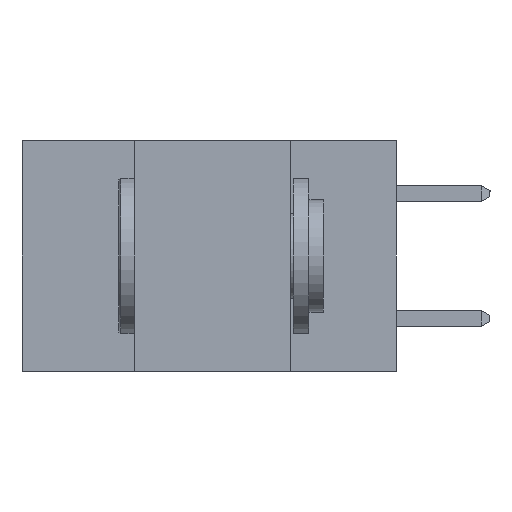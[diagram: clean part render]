
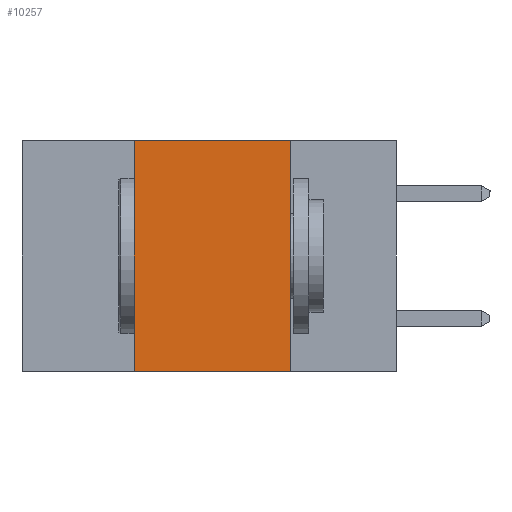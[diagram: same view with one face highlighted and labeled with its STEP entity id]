
A CAD part, left-side view. The second image highlights one B-rep face of the part: STEP entity #10257.
In plain terms, the highlighted planar face has unit normal (-1, 0, 0).
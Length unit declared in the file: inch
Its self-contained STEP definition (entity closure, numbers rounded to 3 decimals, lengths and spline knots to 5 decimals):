
#478 = CARTESIAN_POINT ( 'NONE',  ( 0., 0.6, -0.37 ) ) ;
#759 = DIRECTION ( 'NONE',  ( 0., 0., -1. ) ) ;
#1165 = LINE ( 'NONE', #14763, #4010 ) ;
#1431 = VERTEX_POINT ( 'NONE', #18993 ) ;
#2068 = ORIENTED_EDGE ( 'NONE', *, *, #12775, .T. ) ;
#2248 = VERTEX_POINT ( 'NONE', #3131 ) ;
#3131 = CARTESIAN_POINT ( 'NONE',  ( 0., 0.42, 0. ) ) ;
#4010 = VECTOR ( 'NONE', #21009, 39.37008 ) ;
#4661 = VECTOR ( 'NONE', #16348, 39.37008 ) ;
#5045 = DIRECTION ( 'NONE',  ( 0., 0., -1. ) ) ;
#5070 = EDGE_CURVE ( 'NONE', #1431, #13845, #5148, .T. ) ;
#5087 = CARTESIAN_POINT ( 'NONE',  ( 0., 0.42, -0.37 ) ) ;
#5148 = LINE ( 'NONE', #16434, #9303 ) ;
#5977 = PLANE ( 'NONE',  #16750 ) ;
#6089 = EDGE_CURVE ( 'NONE', #10722, #2248, #13156, .T. ) ;
#8229 = DIRECTION ( 'NONE',  ( 0., 0., 1. ) ) ;
#8542 = EDGE_LOOP ( 'NONE', ( #10098, #16438, #9071, #2068 ) ) ;
#8891 = FACE_OUTER_BOUND ( 'NONE', #8542, .T. ) ;
#8998 = DIRECTION ( 'NONE',  ( 1., 0., 0. ) ) ;
#9071 = ORIENTED_EDGE ( 'NONE', *, *, #6089, .F. ) ;
#9303 = VECTOR ( 'NONE', #5045, 39.37008 ) ;
#10098 = ORIENTED_EDGE ( 'NONE', *, *, #5070, .F. ) ;
#10257 = ADVANCED_FACE ( 'NONE', ( #8891 ), #5977, .F. ) ;
#10722 = VERTEX_POINT ( 'NONE', #14125 ) ;
#12775 = EDGE_CURVE ( 'NONE', #10722, #13845, #13554, .T. ) ;
#13156 = LINE ( 'NONE', #5087, #14172 ) ;
#13554 = LINE ( 'NONE', #478, #4661 ) ;
#13845 = VERTEX_POINT ( 'NONE', #15716 ) ;
#14125 = CARTESIAN_POINT ( 'NONE',  ( 0., 0.42, -0.37 ) ) ;
#14172 = VECTOR ( 'NONE', #8229, 39.37008 ) ;
#14763 = CARTESIAN_POINT ( 'NONE',  ( 0., 0.6, 0. ) ) ;
#14852 = EDGE_CURVE ( 'NONE', #2248, #1431, #1165, .T. ) ;
#15716 = CARTESIAN_POINT ( 'NONE',  ( 0., 0.17, -0.37 ) ) ;
#16348 = DIRECTION ( 'NONE',  ( 0., -1., 0. ) ) ;
#16434 = CARTESIAN_POINT ( 'NONE',  ( 0., 0.17, -0.37 ) ) ;
#16438 = ORIENTED_EDGE ( 'NONE', *, *, #14852, .F. ) ;
#16750 = AXIS2_PLACEMENT_3D ( 'NONE', #18757, #8998, #759 ) ;
#18757 = CARTESIAN_POINT ( 'NONE',  ( 0., 0.6, 0. ) ) ;
#18993 = CARTESIAN_POINT ( 'NONE',  ( 0., 0.17, 0. ) ) ;
#21009 = DIRECTION ( 'NONE',  ( 0., -1., 0. ) ) ;
